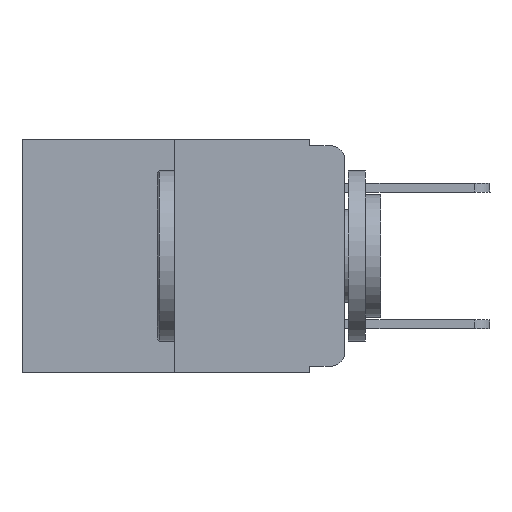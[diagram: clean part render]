
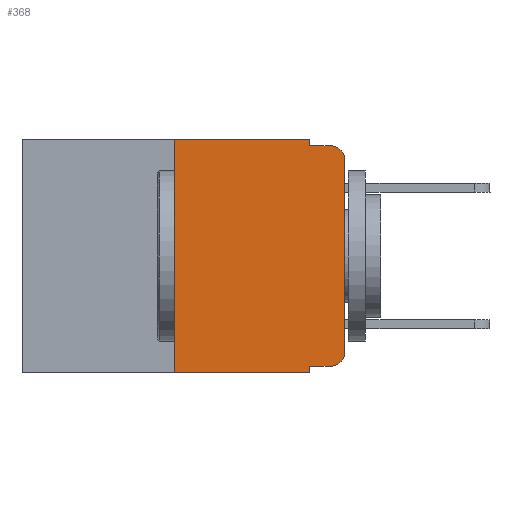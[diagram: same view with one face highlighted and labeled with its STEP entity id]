
A CAD part, left-side view. The second image highlights one B-rep face of the part: STEP entity #368.
In plain terms, the highlighted planar face has unit normal (-1, 0, 0).
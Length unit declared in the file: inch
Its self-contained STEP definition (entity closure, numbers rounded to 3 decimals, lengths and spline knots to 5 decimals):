
#368 = ADVANCED_FACE ( 'NONE', ( #8298 ), #6007, .F. ) ;
#636 = VERTEX_POINT ( 'NONE', #9086 ) ;
#734 = ORIENTED_EDGE ( 'NONE', *, *, #7387, .F. ) ;
#983 = VECTOR ( 'NONE', #10980, 39.37008 ) ;
#997 = ORIENTED_EDGE ( 'NONE', *, *, #12469, .F. ) ;
#1100 = CIRCLE ( 'NONE', #19842, 0.02 ) ;
#1379 = LINE ( 'NONE', #15156, #3608 ) ;
#1509 = VECTOR ( 'NONE', #13852, 39.37008 ) ;
#1637 = ORIENTED_EDGE ( 'NONE', *, *, #17394, .T. ) ;
#2031 = ORIENTED_EDGE ( 'NONE', *, *, #4377, .F. ) ;
#2088 = CARTESIAN_POINT ( 'NONE',  ( 0., 0.051, -0.01 ) ) ;
#2140 = AXIS2_PLACEMENT_3D ( 'NONE', #11842, #19537, #18015 ) ;
#2858 = DIRECTION ( 'NONE',  ( 0., 0., 1. ) ) ;
#3343 = ORIENTED_EDGE ( 'NONE', *, *, #15373, .F. ) ;
#3376 = VECTOR ( 'NONE', #18825, 39.37008 ) ;
#3500 = ORIENTED_EDGE ( 'NONE', *, *, #12894, .F. ) ;
#3544 = CARTESIAN_POINT ( 'NONE',  ( 0., 0.051, -0.01 ) ) ;
#3608 = VECTOR ( 'NONE', #10375, 39.37008 ) ;
#4377 = EDGE_CURVE ( 'NONE', #636, #16724, #4816, .T. ) ;
#4472 = VERTEX_POINT ( 'NONE', #14742 ) ;
#4517 = CARTESIAN_POINT ( 'NONE',  ( 0., 0.051, 0. ) ) ;
#4711 = LINE ( 'NONE', #19922, #1509 ) ;
#4816 = LINE ( 'NONE', #4517, #983 ) ;
#4939 = DIRECTION ( 'NONE',  ( -1., 0., 0. ) ) ;
#5312 = CARTESIAN_POINT ( 'NONE',  ( 0., 0.25, 0. ) ) ;
#5584 = CARTESIAN_POINT ( 'NONE',  ( 0., 0.051, 0. ) ) ;
#5588 = CARTESIAN_POINT ( 'NONE',  ( 0., 0.25, -0.343 ) ) ;
#5653 = VECTOR ( 'NONE', #19302, 39.37008 ) ;
#5708 = EDGE_CURVE ( 'NONE', #10212, #16724, #4711, .T. ) ;
#6007 = PLANE ( 'NONE',  #13090 ) ;
#6727 = EDGE_CURVE ( 'NONE', #14061, #4472, #1100, .T. ) ;
#7065 = LINE ( 'NONE', #13122, #5653 ) ;
#7387 = EDGE_CURVE ( 'NONE', #8136, #12725, #7450, .T. ) ;
#7450 = LINE ( 'NONE', #13624, #8484 ) ;
#8136 = VERTEX_POINT ( 'NONE', #5584 ) ;
#8205 = VERTEX_POINT ( 'NONE', #10421 ) ;
#8247 = EDGE_CURVE ( 'NONE', #12988, #14061, #15307, .T. ) ;
#8268 = CIRCLE ( 'NONE', #2140, 0.02 ) ;
#8298 = FACE_OUTER_BOUND ( 'NONE', #10087, .T. ) ;
#8356 = LINE ( 'NONE', #5312, #18827 ) ;
#8455 = DIRECTION ( 'NONE',  ( 0., 0., 1. ) ) ;
#8484 = VECTOR ( 'NONE', #19902, 39.37008 ) ;
#8603 = DIRECTION ( 'NONE',  ( 1., 0., 0. ) ) ;
#9007 = CARTESIAN_POINT ( 'NONE',  ( 0., 0.051, -0.343 ) ) ;
#9086 = CARTESIAN_POINT ( 'NONE',  ( 0., 0.051, -0.333 ) ) ;
#9800 = LINE ( 'NONE', #3544, #3376 ) ;
#10087 = EDGE_LOOP ( 'NONE', ( #12107, #14025, #3343, #734, #997, #3500, #11580, #2031, #1637, #16187 ) ) ;
#10212 = VERTEX_POINT ( 'NONE', #5588 ) ;
#10298 = DIRECTION ( 'NONE',  ( 0., 0., -1. ) ) ;
#10375 = DIRECTION ( 'NONE',  ( 0., -1., 0. ) ) ;
#10421 = CARTESIAN_POINT ( 'NONE',  ( 0., 0.25, 0. ) ) ;
#10980 = DIRECTION ( 'NONE',  ( 0., 0., -1. ) ) ;
#11111 = DIRECTION ( 'NONE',  ( 0., 0., -1. ) ) ;
#11580 = ORIENTED_EDGE ( 'NONE', *, *, #5708, .T. ) ;
#11842 = CARTESIAN_POINT ( 'NONE',  ( 0., 0.02, -0.313 ) ) ;
#12107 = ORIENTED_EDGE ( 'NONE', *, *, #8247, .T. ) ;
#12188 = CARTESIAN_POINT ( 'NONE',  ( 0., 0.473, 0. ) ) ;
#12469 = EDGE_CURVE ( 'NONE', #8205, #8136, #1379, .T. ) ;
#12664 = CARTESIAN_POINT ( 'NONE',  ( 0., 0.02, -0.03 ) ) ;
#12725 = VERTEX_POINT ( 'NONE', #2088 ) ;
#12894 = EDGE_CURVE ( 'NONE', #10212, #8205, #8356, .T. ) ;
#12988 = VERTEX_POINT ( 'NONE', #13409 ) ;
#13000 = CARTESIAN_POINT ( 'NONE',  ( 0., 0.02, -0.333 ) ) ;
#13090 = AXIS2_PLACEMENT_3D ( 'NONE', #12188, #8603, #10298 ) ;
#13122 = CARTESIAN_POINT ( 'NONE',  ( 0., 0.051, -0.333 ) ) ;
#13409 = CARTESIAN_POINT ( 'NONE',  ( 0., 0., -0.313 ) ) ;
#13624 = CARTESIAN_POINT ( 'NONE',  ( 0., 0.051, 0. ) ) ;
#13852 = DIRECTION ( 'NONE',  ( 0., -1., 0. ) ) ;
#14025 = ORIENTED_EDGE ( 'NONE', *, *, #6727, .T. ) ;
#14061 = VERTEX_POINT ( 'NONE', #18897 ) ;
#14645 = VERTEX_POINT ( 'NONE', #13000 ) ;
#14742 = CARTESIAN_POINT ( 'NONE',  ( 0., 0.02, -0.01 ) ) ;
#14843 = VECTOR ( 'NONE', #2858, 39.37008 ) ;
#15156 = CARTESIAN_POINT ( 'NONE',  ( 0., 0.473, 0. ) ) ;
#15307 = LINE ( 'NONE', #18140, #14843 ) ;
#15373 = EDGE_CURVE ( 'NONE', #12725, #4472, #9800, .T. ) ;
#16187 = ORIENTED_EDGE ( 'NONE', *, *, #18583, .T. ) ;
#16724 = VERTEX_POINT ( 'NONE', #9007 ) ;
#17394 = EDGE_CURVE ( 'NONE', #636, #14645, #7065, .T. ) ;
#18015 = DIRECTION ( 'NONE',  ( 0., 0., -1. ) ) ;
#18140 = CARTESIAN_POINT ( 'NONE',  ( 0., 0., 0. ) ) ;
#18583 = EDGE_CURVE ( 'NONE', #14645, #12988, #8268, .T. ) ;
#18825 = DIRECTION ( 'NONE',  ( 0., -1., 0. ) ) ;
#18827 = VECTOR ( 'NONE', #8455, 39.37008 ) ;
#18897 = CARTESIAN_POINT ( 'NONE',  ( 0., 0., -0.03 ) ) ;
#19302 = DIRECTION ( 'NONE',  ( 0., -1., 0. ) ) ;
#19537 = DIRECTION ( 'NONE',  ( -1., 0., 0. ) ) ;
#19842 = AXIS2_PLACEMENT_3D ( 'NONE', #12664, #4939, #11111 ) ;
#19902 = DIRECTION ( 'NONE',  ( 0., 0., -1. ) ) ;
#19922 = CARTESIAN_POINT ( 'NONE',  ( 0., 0.473, -0.343 ) ) ;
